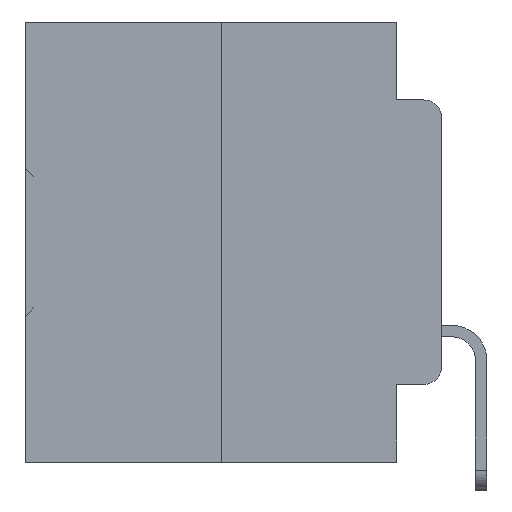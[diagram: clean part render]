
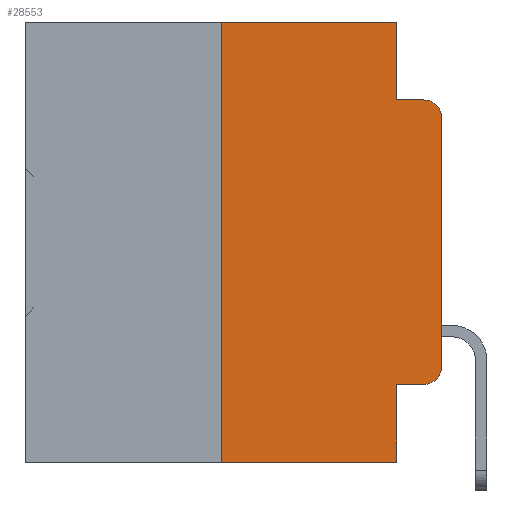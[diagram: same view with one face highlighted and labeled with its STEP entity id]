
A CAD part, left-side view. The second image highlights one B-rep face of the part: STEP entity #28553.
In plain terms, the highlighted planar face has unit normal (-1, 0, 0).
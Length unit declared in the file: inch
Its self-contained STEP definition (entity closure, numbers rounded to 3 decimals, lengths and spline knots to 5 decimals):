
#269 = VERTEX_POINT ( 'NONE', #8193 ) ;
#729 = DIRECTION ( 'NONE',  ( 0., 0., 1. ) ) ;
#826 = CARTESIAN_POINT ( 'NONE',  ( 0., 0.051, -0.0885 ) ) ;
#2467 = EDGE_CURVE ( 'NONE', #24165, #20461, #6648, .T. ) ;
#3215 = CARTESIAN_POINT ( 'NONE',  ( 0., 0.02, -0.0885 ) ) ;
#3923 = CARTESIAN_POINT ( 'NONE',  ( 0., 0.02, -0.1085 ) ) ;
#4187 = DIRECTION ( 'NONE',  ( 0., 0., 1. ) ) ;
#4289 = DIRECTION ( 'NONE',  ( 0., -1., 0. ) ) ;
#4314 = ORIENTED_EDGE ( 'NONE', *, *, #28112, .T. ) ;
#4746 = VECTOR ( 'NONE', #4187, 39.37008 ) ;
#5471 = VERTEX_POINT ( 'NONE', #20559 ) ;
#5520 = CARTESIAN_POINT ( 'NONE',  ( 0., 0.02, -0.3915 ) ) ;
#6648 = LINE ( 'NONE', #34780, #20044 ) ;
#6825 = VECTOR ( 'NONE', #9124, 39.37008 ) ;
#6867 = DIRECTION ( 'NONE',  ( 0., 0., -1. ) ) ;
#7066 = CIRCLE ( 'NONE', #9457, 0.02 ) ;
#7379 = ORIENTED_EDGE ( 'NONE', *, *, #11541, .T. ) ;
#7753 = VERTEX_POINT ( 'NONE', #30521 ) ;
#8193 = CARTESIAN_POINT ( 'NONE',  ( 0., 0.25, 0. ) ) ;
#8462 = DIRECTION ( 'NONE',  ( 0., 0., -1. ) ) ;
#8572 = VECTOR ( 'NONE', #17233, 39.37008 ) ;
#9124 = DIRECTION ( 'NONE',  ( 0., 0., -1. ) ) ;
#9457 = AXIS2_PLACEMENT_3D ( 'NONE', #3923, #23860, #6867 ) ;
#10931 = CARTESIAN_POINT ( 'NONE',  ( 0., 0.051, -0.4115 ) ) ;
#11532 = ORIENTED_EDGE ( 'NONE', *, *, #2467, .T. ) ;
#11541 = EDGE_CURVE ( 'NONE', #5471, #14089, #30936, .T. ) ;
#12358 = CIRCLE ( 'NONE', #22435, 0.02 ) ;
#12887 = EDGE_CURVE ( 'NONE', #20461, #21694, #7066, .T. ) ;
#12979 = LINE ( 'NONE', #18445, #34396 ) ;
#13333 = LINE ( 'NONE', #24080, #4746 ) ;
#14089 = VERTEX_POINT ( 'NONE', #17499 ) ;
#14134 = ORIENTED_EDGE ( 'NONE', *, *, #12887, .T. ) ;
#14279 = EDGE_CURVE ( 'NONE', #5471, #269, #13333, .T. ) ;
#14483 = LINE ( 'NONE', #24351, #21121 ) ;
#14547 = VERTEX_POINT ( 'NONE', #36340 ) ;
#15775 = ORIENTED_EDGE ( 'NONE', *, *, #34198, .F. ) ;
#16316 = VERTEX_POINT ( 'NONE', #10931 ) ;
#16390 = ORIENTED_EDGE ( 'NONE', *, *, #14279, .F. ) ;
#16899 = ORIENTED_EDGE ( 'NONE', *, *, #27449, .F. ) ;
#17233 = DIRECTION ( 'NONE',  ( 0., -1., 0. ) ) ;
#17499 = CARTESIAN_POINT ( 'NONE',  ( 0., 0.051, -0.5 ) ) ;
#18113 = DIRECTION ( 'NONE',  ( 0., 0., -1. ) ) ;
#18445 = CARTESIAN_POINT ( 'NONE',  ( 0., 0.473, 0. ) ) ;
#18779 = EDGE_CURVE ( 'NONE', #14547, #24165, #12358, .T. ) ;
#18952 = ORIENTED_EDGE ( 'NONE', *, *, #18779, .T. ) ;
#19253 = VERTEX_POINT ( 'NONE', #34027 ) ;
#19319 = LINE ( 'NONE', #826, #34111 ) ;
#19999 = LINE ( 'NONE', #35435, #27388 ) ;
#20044 = VECTOR ( 'NONE', #729, 39.37008 ) ;
#20461 = VERTEX_POINT ( 'NONE', #28685 ) ;
#20559 = CARTESIAN_POINT ( 'NONE',  ( 0., 0.25, -0.5 ) ) ;
#21121 = VECTOR ( 'NONE', #21582, 39.37008 ) ;
#21182 = ORIENTED_EDGE ( 'NONE', *, *, #33726, .F. ) ;
#21582 = DIRECTION ( 'NONE',  ( 0., 0., -1. ) ) ;
#21694 = VERTEX_POINT ( 'NONE', #3215 ) ;
#22435 = AXIS2_PLACEMENT_3D ( 'NONE', #5520, #25357, #8462 ) ;
#22560 = ORIENTED_EDGE ( 'NONE', *, *, #25569, .F. ) ;
#23860 = DIRECTION ( 'NONE',  ( -1., 0., 0. ) ) ;
#24080 = CARTESIAN_POINT ( 'NONE',  ( 0., 0.25, 0. ) ) ;
#24165 = VERTEX_POINT ( 'NONE', #33877 ) ;
#24351 = CARTESIAN_POINT ( 'NONE',  ( 0., 0.051, 0. ) ) ;
#25357 = DIRECTION ( 'NONE',  ( -1., 0., 0. ) ) ;
#25569 = EDGE_CURVE ( 'NONE', #19253, #7753, #34983, .T. ) ;
#26405 = PLANE ( 'NONE',  #34943 ) ;
#27388 = VECTOR ( 'NONE', #29811, 39.37008 ) ;
#27449 = EDGE_CURVE ( 'NONE', #269, #19253, #12979, .T. ) ;
#28112 = EDGE_CURVE ( 'NONE', #16316, #14547, #19999, .T. ) ;
#28217 = FACE_OUTER_BOUND ( 'NONE', #33605, .T. ) ;
#28553 = ADVANCED_FACE ( 'NONE', ( #28217 ), #26405, .F. ) ;
#28685 = CARTESIAN_POINT ( 'NONE',  ( 0., 0., -0.1085 ) ) ;
#28757 = CARTESIAN_POINT ( 'NONE',  ( 0., 0.051, 0. ) ) ;
#29150 = CARTESIAN_POINT ( 'NONE',  ( 0., 0.473, 0. ) ) ;
#29811 = DIRECTION ( 'NONE',  ( 0., -1., 0. ) ) ;
#30521 = CARTESIAN_POINT ( 'NONE',  ( 0., 0.051, -0.0885 ) ) ;
#30936 = LINE ( 'NONE', #36691, #8572 ) ;
#31949 = DIRECTION ( 'NONE',  ( 0., -1., 0. ) ) ;
#33605 = EDGE_LOOP ( 'NONE', ( #11532, #14134, #15775, #22560, #16899, #16390, #7379, #21182, #4314, #18952 ) ) ;
#33726 = EDGE_CURVE ( 'NONE', #16316, #14089, #14483, .T. ) ;
#33877 = CARTESIAN_POINT ( 'NONE',  ( 0., 0., -0.3915 ) ) ;
#34027 = CARTESIAN_POINT ( 'NONE',  ( 0., 0.051, 0. ) ) ;
#34111 = VECTOR ( 'NONE', #31949, 39.37008 ) ;
#34198 = EDGE_CURVE ( 'NONE', #7753, #21694, #19319, .T. ) ;
#34396 = VECTOR ( 'NONE', #4289, 39.37008 ) ;
#34780 = CARTESIAN_POINT ( 'NONE',  ( 0., 0., 0. ) ) ;
#34783 = DIRECTION ( 'NONE',  ( 1., 0., 0. ) ) ;
#34943 = AXIS2_PLACEMENT_3D ( 'NONE', #29150, #34783, #18113 ) ;
#34983 = LINE ( 'NONE', #28757, #6825 ) ;
#35435 = CARTESIAN_POINT ( 'NONE',  ( 0., 0.051, -0.4115 ) ) ;
#36340 = CARTESIAN_POINT ( 'NONE',  ( 0., 0.02, -0.4115 ) ) ;
#36691 = CARTESIAN_POINT ( 'NONE',  ( 0., 0.473, -0.5 ) ) ;
